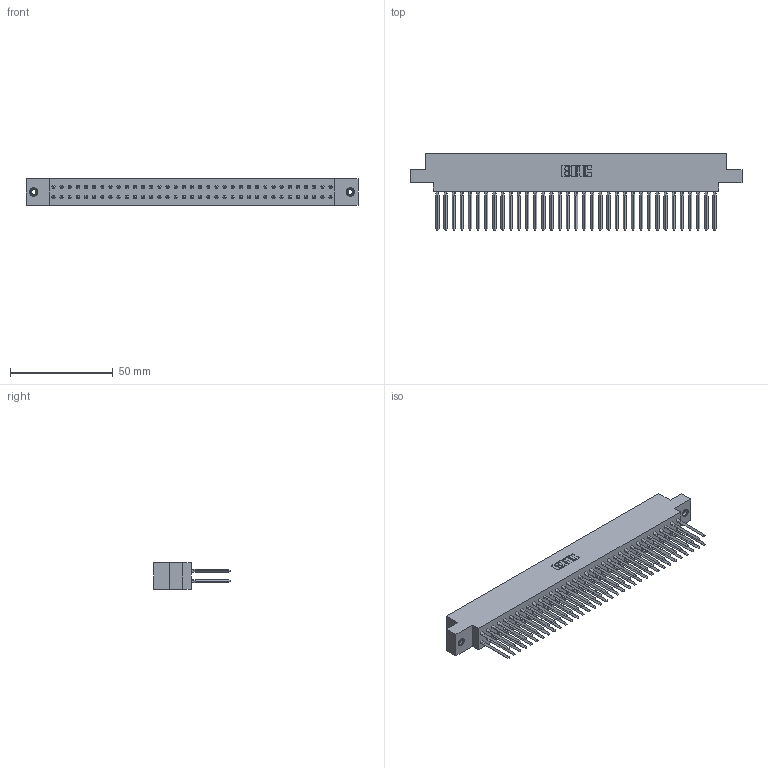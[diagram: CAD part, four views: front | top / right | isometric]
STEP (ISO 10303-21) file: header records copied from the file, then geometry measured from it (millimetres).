
FILE_DESCRIPTION (( 'STEP AP203' ), '1' );
FILE_NAME ('317-070-542-878.STEP', '2020-02-28T07:11:31', ( '' ), ( '' ), 'SwSTEP 2.0', 'SolidWorks 2016', '' );
FILE_SCHEMA (( 'CONFIG_CONTROL_DESIGN' ));
Length unit declared in the file: inch
Products named in the file (4): 317-290-003_542; 345-250-001_345-250-003-102; 317 Part_.156 Dia - TI; 317-070-542-878
Assembly tree (73 placements, depth 2):
  317-070-542-878
    317 Part_.156 Dia - TI
    317-290-003_542  x70
    345-250-001_345-250-003-102  x2
Bounding box: 161.39 x 37.34 x 12.7 mm (x, y, z)
Volume: 26199.6 mm3; surface area: 36230.8 mm2
Topology: 73 solids, 73 shells, 4152 faces, 11611 edges, 7406 vertices
Faces by surface type: plane 3310, cylinder 546, bspline 280, cone 12, torus 4
Entity records: 51772 total; most frequent: CARTESIAN_POINT 9252, ORIENTED_EDGE 8908, DIRECTION 7544, EDGE_CURVE 4454, LINE 4264, VECTOR 4264, VERTEX_POINT 2960, AXIS2_PLACEMENT_3D 1640
